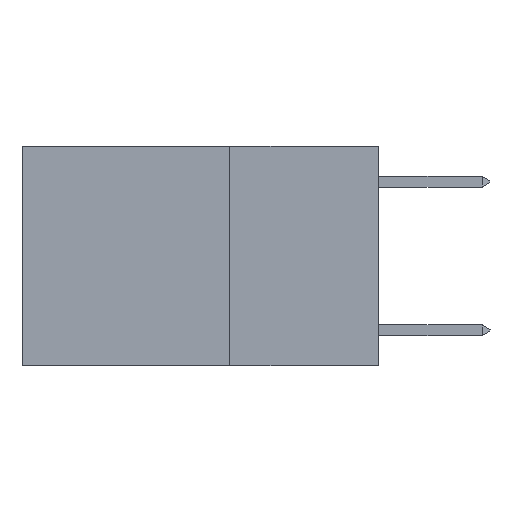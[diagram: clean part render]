
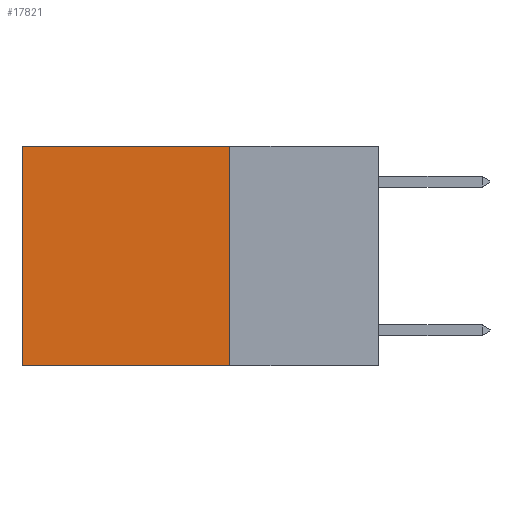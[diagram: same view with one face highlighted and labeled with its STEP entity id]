
A CAD part, left-side view. The second image highlights one B-rep face of the part: STEP entity #17821.
In plain terms, the highlighted planar face has unit normal (-1, 0, 0).
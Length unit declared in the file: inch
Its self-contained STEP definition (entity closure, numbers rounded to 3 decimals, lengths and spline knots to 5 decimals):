
#989 = CARTESIAN_POINT ( 'NONE',  ( 0.2625, 0.25, 0. ) ) ;
#1034 = DIRECTION ( 'NONE',  ( 0., 0., -1. ) ) ;
#1293 = ORIENTED_EDGE ( 'NONE', *, *, #17669, .F. ) ;
#1915 = AXIS2_PLACEMENT_3D ( 'NONE', #19804, #19775, #19569 ) ;
#2230 = EDGE_CURVE ( 'NONE', #10953, #9400, #11006, .T. ) ;
#2317 = DIRECTION ( 'NONE',  ( 0., 1., 0. ) ) ;
#2351 = CARTESIAN_POINT ( 'NONE',  ( 0.2625, 0.25, 0. ) ) ;
#2388 = VECTOR ( 'NONE', #5888, 39.37008 ) ;
#2553 = LINE ( 'NONE', #5542, #2388 ) ;
#3654 = VERTEX_POINT ( 'NONE', #10444 ) ;
#4962 = EDGE_LOOP ( 'NONE', ( #5203, #8692, #1293, #7348 ) ) ;
#5203 = ORIENTED_EDGE ( 'NONE', *, *, #2230, .T. ) ;
#5542 = CARTESIAN_POINT ( 'NONE',  ( 0.2625, 0.25, -0.37 ) ) ;
#5888 = DIRECTION ( 'NONE',  ( 0., 1., 0. ) ) ;
#5972 = FACE_OUTER_BOUND ( 'NONE', #4962, .T. ) ;
#6220 = DIRECTION ( 'NONE',  ( 0., 0., -1. ) ) ;
#7348 = ORIENTED_EDGE ( 'NONE', *, *, #13427, .T. ) ;
#7488 = VECTOR ( 'NONE', #1034, 39.37008 ) ;
#7692 = LINE ( 'NONE', #989, #7488 ) ;
#7804 = CARTESIAN_POINT ( 'NONE',  ( 0.2625, 0.6, 0. ) ) ;
#8692 = ORIENTED_EDGE ( 'NONE', *, *, #15410, .F. ) ;
#9400 = VERTEX_POINT ( 'NONE', #20702 ) ;
#10444 = CARTESIAN_POINT ( 'NONE',  ( 0.2625, 0.25, 0. ) ) ;
#10448 = CARTESIAN_POINT ( 'NONE',  ( 0.2625, 0.6, 0. ) ) ;
#10474 = VECTOR ( 'NONE', #6220, 39.37008 ) ;
#10953 = VERTEX_POINT ( 'NONE', #10448 ) ;
#11006 = LINE ( 'NONE', #7804, #10474 ) ;
#13379 = CARTESIAN_POINT ( 'NONE',  ( 0.2625, 0.25, -0.37 ) ) ;
#13427 = EDGE_CURVE ( 'NONE', #3654, #10953, #13797, .T. ) ;
#13797 = LINE ( 'NONE', #2351, #13903 ) ;
#13903 = VECTOR ( 'NONE', #2317, 39.37008 ) ;
#15410 = EDGE_CURVE ( 'NONE', #18053, #9400, #2553, .T. ) ;
#17669 = EDGE_CURVE ( 'NONE', #3654, #18053, #7692, .T. ) ;
#17821 = ADVANCED_FACE ( 'NONE', ( #5972 ), #21108, .F. ) ;
#18053 = VERTEX_POINT ( 'NONE', #13379 ) ;
#19569 = DIRECTION ( 'NONE',  ( 0., 0., -1. ) ) ;
#19775 = DIRECTION ( 'NONE',  ( 1., 0., 0. ) ) ;
#19804 = CARTESIAN_POINT ( 'NONE',  ( 0.2625, 0.25, 0. ) ) ;
#20702 = CARTESIAN_POINT ( 'NONE',  ( 0.2625, 0.6, -0.37 ) ) ;
#21108 = PLANE ( 'NONE',  #1915 ) ;
